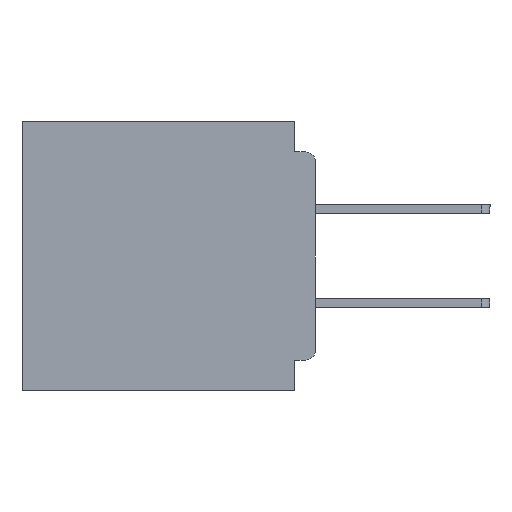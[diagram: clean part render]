
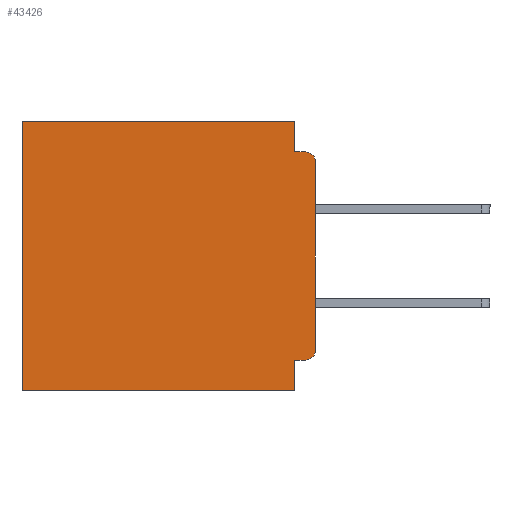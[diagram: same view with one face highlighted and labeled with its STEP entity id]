
A CAD part, left-side view. The second image highlights one B-rep face of the part: STEP entity #43426.
In plain terms, the highlighted planar face has unit normal (-1, 0, 0).
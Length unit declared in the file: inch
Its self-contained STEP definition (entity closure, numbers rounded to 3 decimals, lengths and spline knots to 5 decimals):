
#20 = VERTEX_POINT ( 'NONE', #47930 ) ;
#156 = LINE ( 'NONE', #50420, #50649 ) ;
#2501 = LINE ( 'NONE', #13423, #46205 ) ;
#2826 = PLANE ( 'NONE',  #11198 ) ;
#3491 = CARTESIAN_POINT ( 'NONE',  ( 0.3, 0.031, -0.355 ) ) ;
#3710 = DIRECTION ( 'NONE',  ( 0., 1., 0. ) ) ;
#4983 = CARTESIAN_POINT ( 'NONE',  ( 0.3, 0., -0.4 ) ) ;
#5530 = VECTOR ( 'NONE', #45337, 39.37008 ) ;
#5823 = CARTESIAN_POINT ( 'NONE',  ( 0.3, 0.031, 0. ) ) ;
#6224 = LINE ( 'NONE', #42418, #36834 ) ;
#7720 = CARTESIAN_POINT ( 'NONE',  ( 0.3, 0., -0.355 ) ) ;
#7869 = EDGE_CURVE ( 'NONE', #47475, #50294, #32646, .T. ) ;
#9122 = ORIENTED_EDGE ( 'NONE', *, *, #26419, .T. ) ;
#10297 = ORIENTED_EDGE ( 'NONE', *, *, #12974, .T. ) ;
#10316 = ORIENTED_EDGE ( 'NONE', *, *, #17363, .F. ) ;
#10859 = DIRECTION ( 'NONE',  ( 0., 0., -1. ) ) ;
#11198 = AXIS2_PLACEMENT_3D ( 'NONE', #30785, #34797, #10859 ) ;
#12974 = EDGE_CURVE ( 'NONE', #20508, #38777, #37384, .T. ) ;
#13406 = CARTESIAN_POINT ( 'NONE',  ( 0.3, 0.437, -0.4 ) ) ;
#13423 = CARTESIAN_POINT ( 'NONE',  ( 0.3, 0.031, 0. ) ) ;
#13652 = DIRECTION ( 'NONE',  ( 0., 0., -1. ) ) ;
#14391 = LINE ( 'NONE', #7720, #34370 ) ;
#14513 = DIRECTION ( 'NONE',  ( 0., 1., 0. ) ) ;
#15455 = ORIENTED_EDGE ( 'NONE', *, *, #42676, .T. ) ;
#15899 = VERTEX_POINT ( 'NONE', #48783 ) ;
#17363 = EDGE_CURVE ( 'NONE', #15899, #50294, #28156, .T. ) ;
#17610 = VECTOR ( 'NONE', #32908, 39.37008 ) ;
#17671 = EDGE_CURVE ( 'NONE', #47475, #33630, #14391, .T. ) ;
#17817 = EDGE_LOOP ( 'NONE', ( #10316, #15455, #46353, #18949, #9122, #10297, #35659, #41848, #35165, #19595 ) ) ;
#18084 = EDGE_CURVE ( 'NONE', #47080, #38777, #6224, .T. ) ;
#18205 = CARTESIAN_POINT ( 'NONE',  ( 0.3, 0.015, -0.34 ) ) ;
#18610 = CARTESIAN_POINT ( 'NONE',  ( 0.3, 0.437, -0.4 ) ) ;
#18949 = ORIENTED_EDGE ( 'NONE', *, *, #48385, .F. ) ;
#19392 = CARTESIAN_POINT ( 'NONE',  ( 0.3, 0.015, -0.06 ) ) ;
#19595 = ORIENTED_EDGE ( 'NONE', *, *, #7869, .T. ) ;
#20508 = VERTEX_POINT ( 'NONE', #22377 ) ;
#22203 = DIRECTION ( 'NONE',  ( 0., 0., -1. ) ) ;
#22377 = CARTESIAN_POINT ( 'NONE',  ( 0.3, 0.437, 0. ) ) ;
#23209 = VERTEX_POINT ( 'NONE', #5823 ) ;
#23394 = DIRECTION ( 'NONE',  ( 0., 0., -1. ) ) ;
#23602 = CARTESIAN_POINT ( 'NONE',  ( 0.3, 0.031, -0.045 ) ) ;
#24641 = EDGE_CURVE ( 'NONE', #27795, #20, #156, .T. ) ;
#26200 = CIRCLE ( 'NONE', #41010, 0.015 ) ;
#26419 = EDGE_CURVE ( 'NONE', #23209, #20508, #33984, .T. ) ;
#27795 = VERTEX_POINT ( 'NONE', #23602 ) ;
#28156 = LINE ( 'NONE', #4983, #17610 ) ;
#29289 = LINE ( 'NONE', #37587, #39901 ) ;
#30785 = CARTESIAN_POINT ( 'NONE',  ( 0.3, 0., -0.4 ) ) ;
#31051 = CARTESIAN_POINT ( 'NONE',  ( 0.3, 0., 0. ) ) ;
#32646 = CIRCLE ( 'NONE', #51493, 0.015 ) ;
#32734 = VECTOR ( 'NONE', #43080, 39.37008 ) ;
#32908 = DIRECTION ( 'NONE',  ( 0., 0., -1. ) ) ;
#33630 = VERTEX_POINT ( 'NONE', #3491 ) ;
#33984 = LINE ( 'NONE', #31051, #32734 ) ;
#34370 = VECTOR ( 'NONE', #3710, 39.37008 ) ;
#34797 = DIRECTION ( 'NONE',  ( 1., 0., 0. ) ) ;
#35088 = EDGE_CURVE ( 'NONE', #33630, #47080, #29289, .T. ) ;
#35165 = ORIENTED_EDGE ( 'NONE', *, *, #17671, .F. ) ;
#35659 = ORIENTED_EDGE ( 'NONE', *, *, #18084, .F. ) ;
#36834 = VECTOR ( 'NONE', #14513, 39.37008 ) ;
#37135 = CARTESIAN_POINT ( 'NONE',  ( 0.3, 0.031, -0.4 ) ) ;
#37362 = DIRECTION ( 'NONE',  ( 0., 0., -1. ) ) ;
#37384 = LINE ( 'NONE', #13406, #5530 ) ;
#37587 = CARTESIAN_POINT ( 'NONE',  ( 0.3, 0.031, -0.4 ) ) ;
#38777 = VERTEX_POINT ( 'NONE', #18610 ) ;
#39901 = VECTOR ( 'NONE', #13652, 39.37008 ) ;
#41010 = AXIS2_PLACEMENT_3D ( 'NONE', #19392, #47224, #23394 ) ;
#41213 = FACE_OUTER_BOUND ( 'NONE', #17817, .T. ) ;
#41848 = ORIENTED_EDGE ( 'NONE', *, *, #35088, .F. ) ;
#42418 = CARTESIAN_POINT ( 'NONE',  ( 0.3, 0., -0.4 ) ) ;
#42676 = EDGE_CURVE ( 'NONE', #15899, #20, #26200, .T. ) ;
#43080 = DIRECTION ( 'NONE',  ( 0., 1., 0. ) ) ;
#43426 = ADVANCED_FACE ( 'NONE', ( #41213 ), #2826, .F. ) ;
#43531 = CARTESIAN_POINT ( 'NONE',  ( 0.3, 0.015, -0.355 ) ) ;
#45337 = DIRECTION ( 'NONE',  ( 0., 0., -1. ) ) ;
#46044 = DIRECTION ( 'NONE',  ( -1., 0., 0. ) ) ;
#46205 = VECTOR ( 'NONE', #37362, 39.37008 ) ;
#46353 = ORIENTED_EDGE ( 'NONE', *, *, #24641, .F. ) ;
#46475 = DIRECTION ( 'NONE',  ( 0., -1., 0. ) ) ;
#47080 = VERTEX_POINT ( 'NONE', #37135 ) ;
#47098 = CARTESIAN_POINT ( 'NONE',  ( 0.3, 0., -0.34 ) ) ;
#47224 = DIRECTION ( 'NONE',  ( -1., 0., 0. ) ) ;
#47475 = VERTEX_POINT ( 'NONE', #43531 ) ;
#47930 = CARTESIAN_POINT ( 'NONE',  ( 0.3, 0.015, -0.045 ) ) ;
#48385 = EDGE_CURVE ( 'NONE', #23209, #27795, #2501, .T. ) ;
#48783 = CARTESIAN_POINT ( 'NONE',  ( 0.3, 0., -0.06 ) ) ;
#50294 = VERTEX_POINT ( 'NONE', #47098 ) ;
#50420 = CARTESIAN_POINT ( 'NONE',  ( 0.3, 0., -0.045 ) ) ;
#50649 = VECTOR ( 'NONE', #46475, 39.37008 ) ;
#51493 = AXIS2_PLACEMENT_3D ( 'NONE', #18205, #46044, #22203 ) ;
